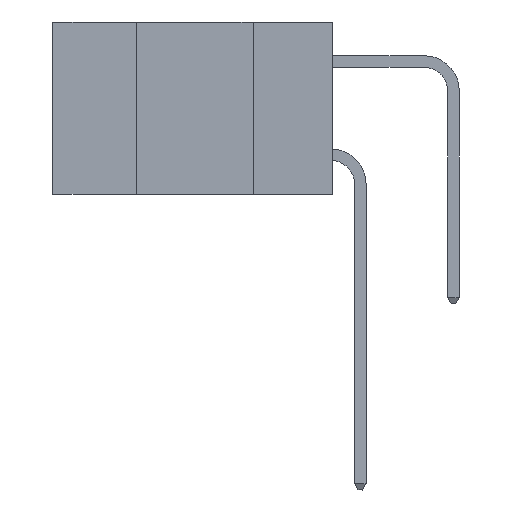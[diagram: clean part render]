
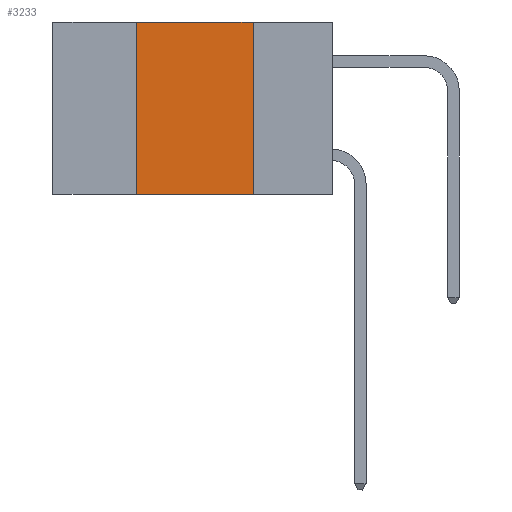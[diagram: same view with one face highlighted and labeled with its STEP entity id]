
A CAD part, left-side view. The second image highlights one B-rep face of the part: STEP entity #3233.
In plain terms, the highlighted planar face has unit normal (-1, 0, 0).
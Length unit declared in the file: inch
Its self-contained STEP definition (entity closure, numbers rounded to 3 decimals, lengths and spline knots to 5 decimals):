
#28 = CARTESIAN_POINT ( 'NONE',  ( 0., 0.6, -0.37 ) ) ;
#158 = ORIENTED_EDGE ( 'NONE', *, *, #2199, .F. ) ;
#2199 = EDGE_CURVE ( 'NONE', #6888, #12989, #6611, .T. ) ;
#2298 = VECTOR ( 'NONE', #8469, 39.37008 ) ;
#2712 = LINE ( 'NONE', #8294, #13674 ) ;
#3233 = ADVANCED_FACE ( 'NONE', ( #13078 ), #5427, .F. ) ;
#3489 = CARTESIAN_POINT ( 'NONE',  ( 0., 0.42, -0.37 ) ) ;
#3800 = VECTOR ( 'NONE', #9158, 39.37008 ) ;
#5372 = DIRECTION ( 'NONE',  ( 1., 0., 0. ) ) ;
#5427 = PLANE ( 'NONE',  #7637 ) ;
#6244 = ORIENTED_EDGE ( 'NONE', *, *, #13128, .T. ) ;
#6281 = DIRECTION ( 'NONE',  ( 0., -1., 0. ) ) ;
#6385 = CARTESIAN_POINT ( 'NONE',  ( 0., 0.6, 0. ) ) ;
#6422 = DIRECTION ( 'NONE',  ( 0., 0., -1. ) ) ;
#6611 = LINE ( 'NONE', #13528, #3800 ) ;
#6888 = VERTEX_POINT ( 'NONE', #3489 ) ;
#7637 = AXIS2_PLACEMENT_3D ( 'NONE', #6385, #5372, #12786 ) ;
#8058 = VERTEX_POINT ( 'NONE', #11606 ) ;
#8089 = ORIENTED_EDGE ( 'NONE', *, *, #9714, .F. ) ;
#8287 = VERTEX_POINT ( 'NONE', #9130 ) ;
#8294 = CARTESIAN_POINT ( 'NONE',  ( 0., 0.6, 0. ) ) ;
#8469 = DIRECTION ( 'NONE',  ( 0., -1., 0. ) ) ;
#9130 = CARTESIAN_POINT ( 'NONE',  ( 0., 0.17, -0.37 ) ) ;
#9158 = DIRECTION ( 'NONE',  ( 0., 0., 1. ) ) ;
#9714 = EDGE_CURVE ( 'NONE', #12989, #8058, #2712, .T. ) ;
#9775 = LINE ( 'NONE', #12594, #12441 ) ;
#10417 = ORIENTED_EDGE ( 'NONE', *, *, #12354, .F. ) ;
#11493 = EDGE_LOOP ( 'NONE', ( #10417, #8089, #158, #6244 ) ) ;
#11606 = CARTESIAN_POINT ( 'NONE',  ( 0., 0.17, 0. ) ) ;
#12354 = EDGE_CURVE ( 'NONE', #8058, #8287, #9775, .T. ) ;
#12441 = VECTOR ( 'NONE', #6422, 39.37008 ) ;
#12594 = CARTESIAN_POINT ( 'NONE',  ( 0., 0.17, 0. ) ) ;
#12786 = DIRECTION ( 'NONE',  ( 0., 0., -1. ) ) ;
#12989 = VERTEX_POINT ( 'NONE', #13596 ) ;
#13078 = FACE_OUTER_BOUND ( 'NONE', #11493, .T. ) ;
#13128 = EDGE_CURVE ( 'NONE', #6888, #8287, #13568, .T. ) ;
#13528 = CARTESIAN_POINT ( 'NONE',  ( 0., 0.42, 0. ) ) ;
#13568 = LINE ( 'NONE', #28, #2298 ) ;
#13596 = CARTESIAN_POINT ( 'NONE',  ( 0., 0.42, 0. ) ) ;
#13674 = VECTOR ( 'NONE', #6281, 39.37008 ) ;
